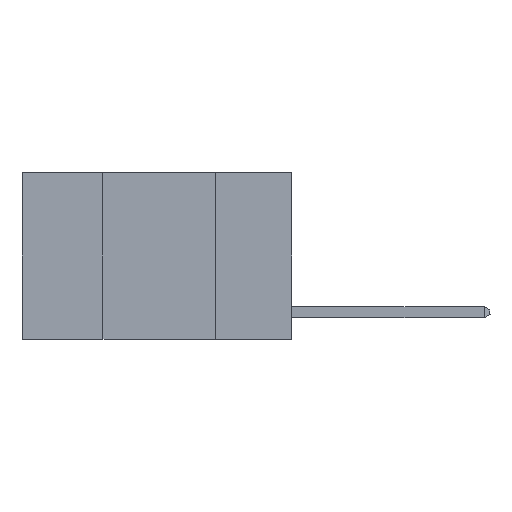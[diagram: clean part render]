
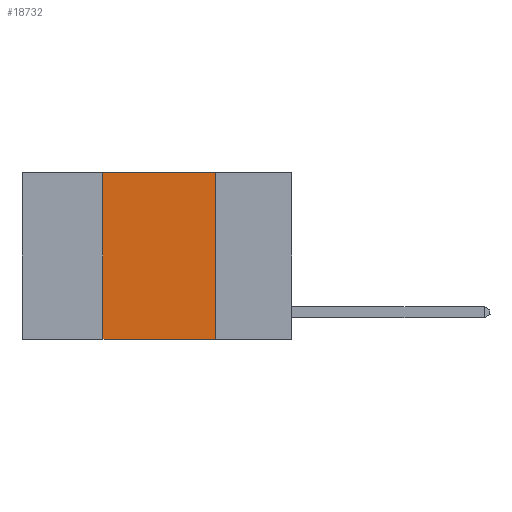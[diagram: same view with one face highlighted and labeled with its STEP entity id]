
A CAD part, left-side view. The second image highlights one B-rep face of the part: STEP entity #18732.
In plain terms, the highlighted planar face has unit normal (-1, 0, 0).
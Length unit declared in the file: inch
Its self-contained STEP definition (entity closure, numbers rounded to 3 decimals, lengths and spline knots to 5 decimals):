
#176 = DIRECTION ( 'NONE',  ( 0., 0., -1. ) ) ;
#1033 = CARTESIAN_POINT ( 'NONE',  ( 0., 0.6, 0. ) ) ;
#1249 = VERTEX_POINT ( 'NONE', #13945 ) ;
#1476 = FACE_OUTER_BOUND ( 'NONE', #22238, .T. ) ;
#1879 = LINE ( 'NONE', #8873, #12635 ) ;
#2529 = VECTOR ( 'NONE', #16641, 39.37008 ) ;
#3881 = VERTEX_POINT ( 'NONE', #17983 ) ;
#4544 = VERTEX_POINT ( 'NONE', #10416 ) ;
#5763 = ORIENTED_EDGE ( 'NONE', *, *, #9547, .T. ) ;
#6971 = CARTESIAN_POINT ( 'NONE',  ( 0., 0.42, -0.37 ) ) ;
#7436 = EDGE_CURVE ( 'NONE', #1249, #4544, #1879, .T. ) ;
#7918 = ORIENTED_EDGE ( 'NONE', *, *, #7436, .F. ) ;
#7955 = VECTOR ( 'NONE', #14432, 39.37008 ) ;
#7988 = LINE ( 'NONE', #14927, #9890 ) ;
#8768 = EDGE_CURVE ( 'NONE', #18832, #3881, #21640, .T. ) ;
#8873 = CARTESIAN_POINT ( 'NONE',  ( 0., 0.17, 0. ) ) ;
#9547 = EDGE_CURVE ( 'NONE', #18832, #4544, #20520, .T. ) ;
#9559 = CARTESIAN_POINT ( 'NONE',  ( 0., 0.42, 0. ) ) ;
#9839 = DIRECTION ( 'NONE',  ( 0., 0., -1. ) ) ;
#9890 = VECTOR ( 'NONE', #13222, 39.37008 ) ;
#10416 = CARTESIAN_POINT ( 'NONE',  ( 0., 0.17, -0.37 ) ) ;
#12635 = VECTOR ( 'NONE', #176, 39.37008 ) ;
#12743 = EDGE_CURVE ( 'NONE', #3881, #1249, #7988, .T. ) ;
#13222 = DIRECTION ( 'NONE',  ( 0., -1., 0. ) ) ;
#13707 = ORIENTED_EDGE ( 'NONE', *, *, #8768, .F. ) ;
#13945 = CARTESIAN_POINT ( 'NONE',  ( 0., 0.17, 0. ) ) ;
#14432 = DIRECTION ( 'NONE',  ( 0., 0., 1. ) ) ;
#14927 = CARTESIAN_POINT ( 'NONE',  ( 0., 0.6, 0. ) ) ;
#15054 = PLANE ( 'NONE',  #16933 ) ;
#16641 = DIRECTION ( 'NONE',  ( 0., -1., 0. ) ) ;
#16933 = AXIS2_PLACEMENT_3D ( 'NONE', #1033, #22041, #9839 ) ;
#17983 = CARTESIAN_POINT ( 'NONE',  ( 0., 0.42, 0. ) ) ;
#18732 = ADVANCED_FACE ( 'NONE', ( #1476 ), #15054, .F. ) ;
#18832 = VERTEX_POINT ( 'NONE', #6971 ) ;
#20520 = LINE ( 'NONE', #22007, #2529 ) ;
#21640 = LINE ( 'NONE', #9559, #7955 ) ;
#22007 = CARTESIAN_POINT ( 'NONE',  ( 0., 0.6, -0.37 ) ) ;
#22041 = DIRECTION ( 'NONE',  ( 1., 0., 0. ) ) ;
#22238 = EDGE_LOOP ( 'NONE', ( #7918, #22367, #13707, #5763 ) ) ;
#22367 = ORIENTED_EDGE ( 'NONE', *, *, #12743, .F. ) ;
